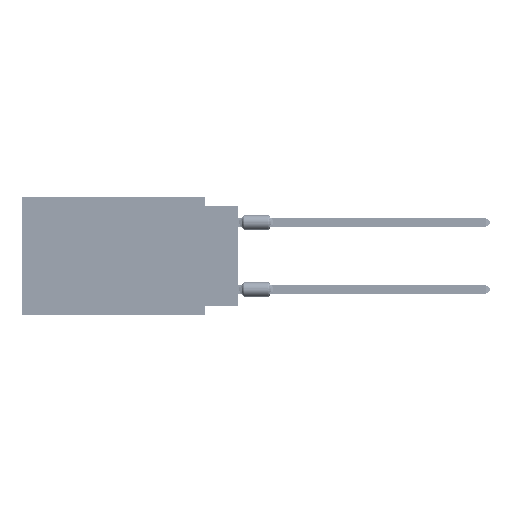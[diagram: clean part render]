
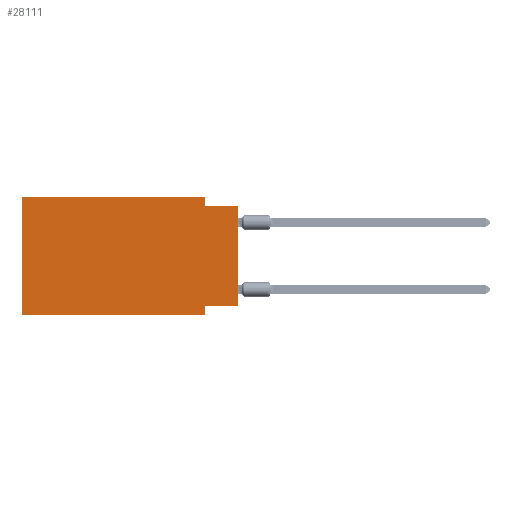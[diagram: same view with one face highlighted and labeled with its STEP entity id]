
A CAD part, left-side view. The second image highlights one B-rep face of the part: STEP entity #28111.
In plain terms, the highlighted planar face has unit normal (-1, 0, 0).
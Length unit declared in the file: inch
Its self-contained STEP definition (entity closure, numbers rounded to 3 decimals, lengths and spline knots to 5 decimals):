
#1152 = VECTOR ( 'NONE', #43933, 39.37008 ) ;
#1364 = DIRECTION ( 'NONE',  ( 0., 0., 1. ) ) ;
#1988 = CARTESIAN_POINT ( 'NONE',  ( 0., 0., -0.325 ) ) ;
#2460 = VECTOR ( 'NONE', #73584, 39.37008 ) ;
#2893 = LINE ( 'NONE', #57985, #53627 ) ;
#3711 = CARTESIAN_POINT ( 'NONE',  ( 0., 0.645, 0. ) ) ;
#6515 = VERTEX_POINT ( 'NONE', #39338 ) ;
#7709 = DIRECTION ( 'NONE',  ( 1., 0., 0. ) ) ;
#8166 = EDGE_CURVE ( 'NONE', #6515, #17567, #37905, .T. ) ;
#10355 = CARTESIAN_POINT ( 'NONE',  ( 0., 0., -0.025 ) ) ;
#10405 = VERTEX_POINT ( 'NONE', #71975 ) ;
#10899 = VECTOR ( 'NONE', #47169, 39.37008 ) ;
#11803 = VECTOR ( 'NONE', #70623, 39.37008 ) ;
#12728 = ORIENTED_EDGE ( 'NONE', *, *, #59385, .F. ) ;
#16011 = DIRECTION ( 'NONE',  ( 0., 0., -1. ) ) ;
#17567 = VERTEX_POINT ( 'NONE', #33417 ) ;
#19303 = ORIENTED_EDGE ( 'NONE', *, *, #81628, .F. ) ;
#21854 = LINE ( 'NONE', #1988, #11803 ) ;
#22367 = EDGE_LOOP ( 'NONE', ( #76871, #61241, #31809, #19303, #76387, #38056, #27954, #12728 ) ) ;
#23032 = CARTESIAN_POINT ( 'NONE',  ( 0., 0., -0.325 ) ) ;
#24859 = EDGE_CURVE ( 'NONE', #10405, #57252, #2893, .T. ) ;
#27954 = ORIENTED_EDGE ( 'NONE', *, *, #24859, .F. ) ;
#28111 = ADVANCED_FACE ( 'NONE', ( #83125 ), #84028, .F. ) ;
#28885 = LINE ( 'NONE', #76773, #64588 ) ;
#31809 = ORIENTED_EDGE ( 'NONE', *, *, #43111, .F. ) ;
#33417 = CARTESIAN_POINT ( 'NONE',  ( 0., 0., -0.025 ) ) ;
#33611 = CARTESIAN_POINT ( 'NONE',  ( 0., 0.645, 0. ) ) ;
#37905 = LINE ( 'NONE', #10355, #77281 ) ;
#38056 = ORIENTED_EDGE ( 'NONE', *, *, #66684, .T. ) ;
#38360 = DIRECTION ( 'NONE',  ( 0., -1., 0. ) ) ;
#39338 = CARTESIAN_POINT ( 'NONE',  ( 0., 0.1, -0.025 ) ) ;
#40850 = LINE ( 'NONE', #41296, #10899 ) ;
#41296 = CARTESIAN_POINT ( 'NONE',  ( 0., 0.645, -0.35 ) ) ;
#43111 = EDGE_CURVE ( 'NONE', #82717, #6515, #51223, .T. ) ;
#43933 = DIRECTION ( 'NONE',  ( 0., -1., 0. ) ) ;
#47169 = DIRECTION ( 'NONE',  ( 0., -1., 0. ) ) ;
#48675 = VECTOR ( 'NONE', #73319, 39.37008 ) ;
#48798 = DIRECTION ( 'NONE',  ( 0., 0., -1. ) ) ;
#49709 = AXIS2_PLACEMENT_3D ( 'NONE', #83564, #7709, #48798 ) ;
#51223 = LINE ( 'NONE', #78779, #48675 ) ;
#53627 = VECTOR ( 'NONE', #16011, 39.37008 ) ;
#56796 = VERTEX_POINT ( 'NONE', #33611 ) ;
#57252 = VERTEX_POINT ( 'NONE', #89050 ) ;
#57985 = CARTESIAN_POINT ( 'NONE',  ( 0., 0.1, -0.35 ) ) ;
#59385 = EDGE_CURVE ( 'NONE', #83325, #10405, #21854, .T. ) ;
#60464 = LINE ( 'NONE', #80362, #2460 ) ;
#61241 = ORIENTED_EDGE ( 'NONE', *, *, #8166, .F. ) ;
#64588 = VECTOR ( 'NONE', #1364, 39.37008 ) ;
#66614 = VERTEX_POINT ( 'NONE', #78826 ) ;
#66684 = EDGE_CURVE ( 'NONE', #66614, #57252, #40850, .T. ) ;
#70623 = DIRECTION ( 'NONE',  ( 0., 1., 0. ) ) ;
#71975 = CARTESIAN_POINT ( 'NONE',  ( 0., 0.1, -0.325 ) ) ;
#73319 = DIRECTION ( 'NONE',  ( 0., 0., -1. ) ) ;
#73584 = DIRECTION ( 'NONE',  ( 0., 0., 1. ) ) ;
#76387 = ORIENTED_EDGE ( 'NONE', *, *, #80146, .F. ) ;
#76462 = CARTESIAN_POINT ( 'NONE',  ( 0., 0.1, 0. ) ) ;
#76773 = CARTESIAN_POINT ( 'NONE',  ( 0., 0.645, 0. ) ) ;
#76871 = ORIENTED_EDGE ( 'NONE', *, *, #83435, .T. ) ;
#77281 = VECTOR ( 'NONE', #38360, 39.37008 ) ;
#78697 = LINE ( 'NONE', #3711, #1152 ) ;
#78779 = CARTESIAN_POINT ( 'NONE',  ( 0., 0.1, 0. ) ) ;
#78826 = CARTESIAN_POINT ( 'NONE',  ( 0., 0.645, -0.35 ) ) ;
#80146 = EDGE_CURVE ( 'NONE', #66614, #56796, #28885, .T. ) ;
#80362 = CARTESIAN_POINT ( 'NONE',  ( 0., 0., 0. ) ) ;
#81628 = EDGE_CURVE ( 'NONE', #56796, #82717, #78697, .T. ) ;
#82717 = VERTEX_POINT ( 'NONE', #76462 ) ;
#83125 = FACE_OUTER_BOUND ( 'NONE', #22367, .T. ) ;
#83325 = VERTEX_POINT ( 'NONE', #23032 ) ;
#83435 = EDGE_CURVE ( 'NONE', #83325, #17567, #60464, .T. ) ;
#83564 = CARTESIAN_POINT ( 'NONE',  ( 0., 0.645, 0. ) ) ;
#84028 = PLANE ( 'NONE',  #49709 ) ;
#89050 = CARTESIAN_POINT ( 'NONE',  ( 0., 0.1, -0.35 ) ) ;
